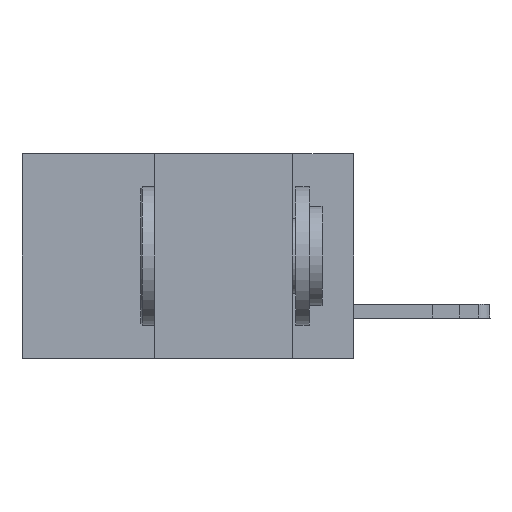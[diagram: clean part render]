
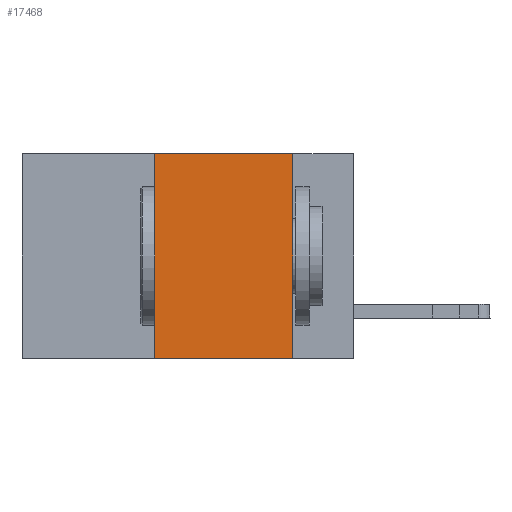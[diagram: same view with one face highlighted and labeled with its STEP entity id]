
A CAD part, left-side view. The second image highlights one B-rep face of the part: STEP entity #17468.
In plain terms, the highlighted planar face has unit normal (-1, 0, 0).
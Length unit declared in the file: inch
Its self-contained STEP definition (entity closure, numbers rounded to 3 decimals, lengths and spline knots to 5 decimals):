
#98 = CARTESIAN_POINT ( 'NONE',  ( 0., 0.6, 0. ) ) ;
#397 = DIRECTION ( 'NONE',  ( 0., 0., -1. ) ) ;
#1039 = DIRECTION ( 'NONE',  ( 0., 0., 1. ) ) ;
#1146 = LINE ( 'NONE', #9154, #12232 ) ;
#1413 = VERTEX_POINT ( 'NONE', #24563 ) ;
#2219 = DIRECTION ( 'NONE',  ( 0., -1., 0. ) ) ;
#5331 = EDGE_CURVE ( 'NONE', #23109, #19815, #11769, .T. ) ;
#6000 = DIRECTION ( 'NONE',  ( 1., 0., 0. ) ) ;
#6189 = CARTESIAN_POINT ( 'NONE',  ( 0., 0.6, 0. ) ) ;
#6926 = AXIS2_PLACEMENT_3D ( 'NONE', #6189, #6000, #8054 ) ;
#8054 = DIRECTION ( 'NONE',  ( 0., 0., -1. ) ) ;
#8362 = EDGE_CURVE ( 'NONE', #23109, #1413, #26856, .T. ) ;
#8401 = VECTOR ( 'NONE', #2219, 39.37008 ) ;
#9154 = CARTESIAN_POINT ( 'NONE',  ( 0., 0.11, 0. ) ) ;
#9330 = EDGE_LOOP ( 'NONE', ( #10291, #24893, #20116, #19386 ) ) ;
#10291 = ORIENTED_EDGE ( 'NONE', *, *, #21202, .F. ) ;
#11769 = LINE ( 'NONE', #17834, #17178 ) ;
#12232 = VECTOR ( 'NONE', #397, 39.37008 ) ;
#13830 = FACE_OUTER_BOUND ( 'NONE', #9330, .T. ) ;
#15165 = EDGE_CURVE ( 'NONE', #1413, #22744, #26288, .T. ) ;
#15320 = VECTOR ( 'NONE', #1039, 39.37008 ) ;
#17178 = VECTOR ( 'NONE', #26650, 39.37008 ) ;
#17468 = ADVANCED_FACE ( 'NONE', ( #13830 ), #27418, .F. ) ;
#17834 = CARTESIAN_POINT ( 'NONE',  ( 0., 0.6, -0.37 ) ) ;
#18089 = CARTESIAN_POINT ( 'NONE',  ( 0., 0.36, 0. ) ) ;
#19386 = ORIENTED_EDGE ( 'NONE', *, *, #5331, .T. ) ;
#19815 = VERTEX_POINT ( 'NONE', #23019 ) ;
#20116 = ORIENTED_EDGE ( 'NONE', *, *, #8362, .F. ) ;
#21202 = EDGE_CURVE ( 'NONE', #22744, #19815, #1146, .T. ) ;
#22435 = CARTESIAN_POINT ( 'NONE',  ( 0., 0.36, -0.37 ) ) ;
#22744 = VERTEX_POINT ( 'NONE', #23329 ) ;
#23019 = CARTESIAN_POINT ( 'NONE',  ( 0., 0.11, -0.37 ) ) ;
#23109 = VERTEX_POINT ( 'NONE', #22435 ) ;
#23329 = CARTESIAN_POINT ( 'NONE',  ( 0., 0.11, 0. ) ) ;
#24563 = CARTESIAN_POINT ( 'NONE',  ( 0., 0.36, 0. ) ) ;
#24893 = ORIENTED_EDGE ( 'NONE', *, *, #15165, .F. ) ;
#26288 = LINE ( 'NONE', #98, #8401 ) ;
#26650 = DIRECTION ( 'NONE',  ( 0., -1., 0. ) ) ;
#26856 = LINE ( 'NONE', #18089, #15320 ) ;
#27418 = PLANE ( 'NONE',  #6926 ) ;
